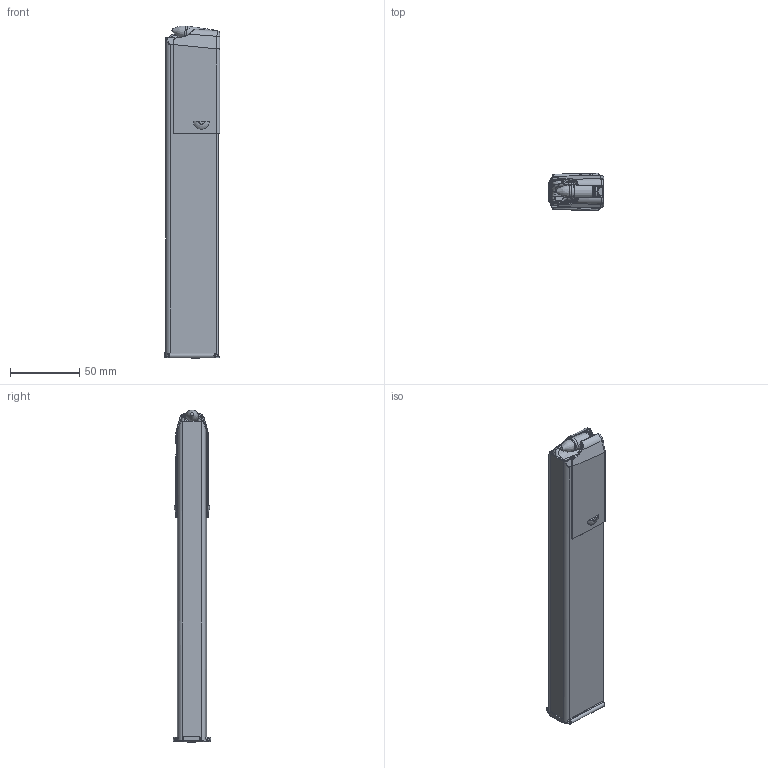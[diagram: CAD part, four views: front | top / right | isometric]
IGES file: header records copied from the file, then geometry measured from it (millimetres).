
Global section: file name: No Iges File Name specified; native system: Autodesk Inventor 2012; preprocessor: AutoDesk Inventor Iges Exporter R2012; author: Michael Høgh; date: 20120201.180034; units: millimetre
Bounding box: 40.06 x 27.39 x 239.84 mm (x, y, z)
Volume: 41830.8 mm3; surface area: 89053.8 mm2
Topology: 9 solids, 9 shells, 819 faces, 1971 edges, 1178 vertices
Faces by surface type: bspline 296, plane 218, cylinder 144, revolution 119, cone 23, torus 15, sphere 4
Full cylindrical faces by diameter (mm): 1.5 x57, 4 x1, 6 x1, 8.79 x1, 9.96 x1
